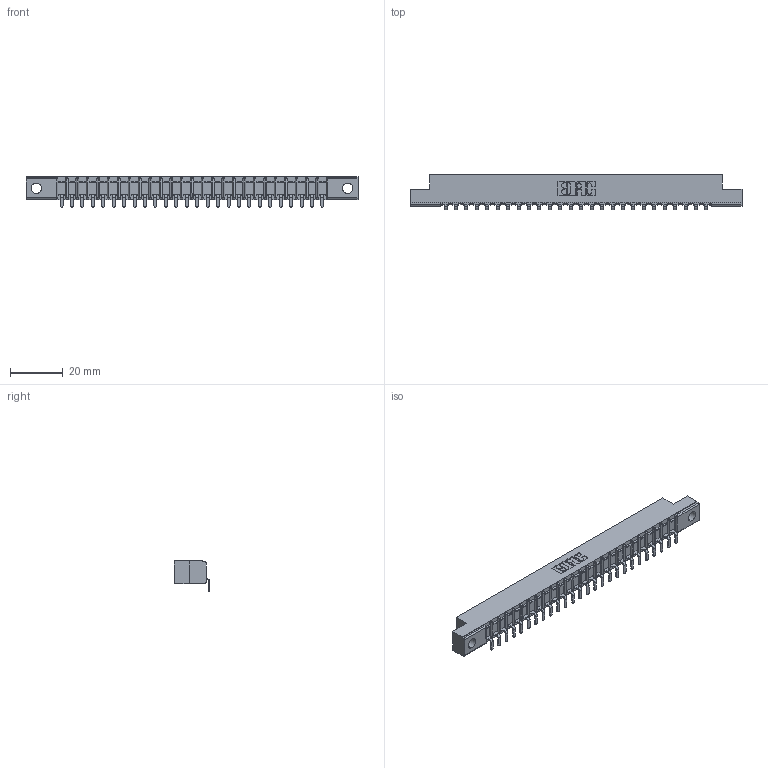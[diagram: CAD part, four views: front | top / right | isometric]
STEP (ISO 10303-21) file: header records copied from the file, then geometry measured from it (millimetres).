
FILE_DESCRIPTION (( 'STEP AP203' ), '1' );
FILE_NAME ('357-026-553-102.STEP', '2018-08-09T03:09:01', ( '' ), ( '' ), 'SwSTEP 2.0', 'SolidWorks 2016', '' );
FILE_SCHEMA (( 'CONFIG_CONTROL_DESIGN' ));
Length unit declared in the file: inch
Products named in the file (3): 307-290-002_553; 357-026-553-102; 307 Part_.128 Dia Mounting Holes
Assembly tree (27 placements, depth 2):
  357-026-553-102
    307 Part_.128 Dia Mounting Holes
    307-290-002_553  x26
Bounding box: 126.03 x 13.32 x 11.51 mm (x, y, z)
Volume: 8234.7 mm3; surface area: 15056 mm2
Topology: 27 solids, 27 shells, 2173 faces, 6667 edges, 4370 vertices
Faces by surface type: plane 1292, cylinder 827, sphere 54
Entity records: 25118 total; most frequent: CARTESIAN_POINT 4236, ORIENTED_EDGE 4226, DIRECTION 4123, EDGE_CURVE 2113, LINE 1609, VECTOR 1609, VERTEX_POINT 1370, AXIS2_PLACEMENT_3D 1257
